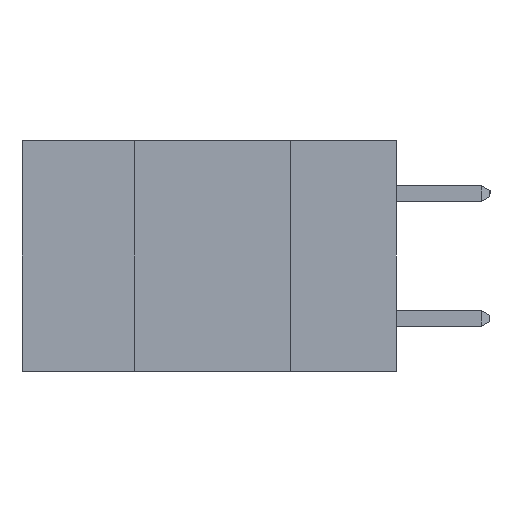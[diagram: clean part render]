
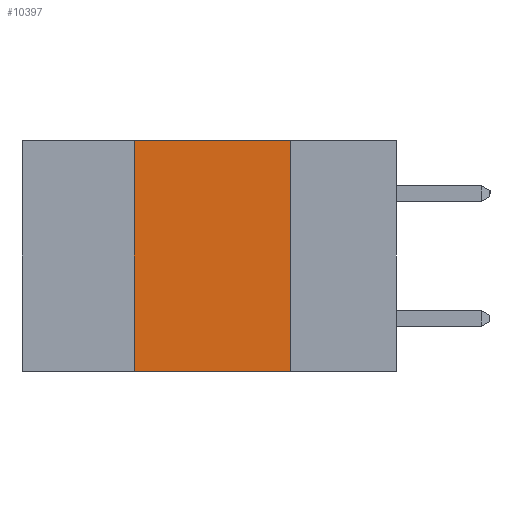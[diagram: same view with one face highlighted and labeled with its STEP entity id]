
A CAD part, left-side view. The second image highlights one B-rep face of the part: STEP entity #10397.
In plain terms, the highlighted planar face has unit normal (-1, 0, 0).
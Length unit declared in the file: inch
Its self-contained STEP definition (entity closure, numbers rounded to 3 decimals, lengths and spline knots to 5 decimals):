
#1438 = PLANE ( 'NONE',  #9139 ) ;
#1587 = EDGE_CURVE ( 'NONE', #10237, #1676, #16990, .T. ) ;
#1663 = FACE_OUTER_BOUND ( 'NONE', #21955, .T. ) ;
#1676 = VERTEX_POINT ( 'NONE', #15715 ) ;
#2738 = ORIENTED_EDGE ( 'NONE', *, *, #1587, .F. ) ;
#3343 = CARTESIAN_POINT ( 'NONE',  ( 0., 0.42, -0.37 ) ) ;
#3896 = VECTOR ( 'NONE', #15156, 39.37008 ) ;
#4046 = VECTOR ( 'NONE', #12525, 39.37008 ) ;
#5323 = CARTESIAN_POINT ( 'NONE',  ( 0., 0.42, -0.37 ) ) ;
#5791 = ORIENTED_EDGE ( 'NONE', *, *, #12398, .T. ) ;
#6889 = DIRECTION ( 'NONE',  ( 0., 0., -1. ) ) ;
#7062 = LINE ( 'NONE', #20868, #15044 ) ;
#9139 = AXIS2_PLACEMENT_3D ( 'NONE', #13674, #20622, #12183 ) ;
#9713 = VERTEX_POINT ( 'NONE', #3343 ) ;
#10237 = VERTEX_POINT ( 'NONE', #16643 ) ;
#10352 = VECTOR ( 'NONE', #6889, 39.37008 ) ;
#10397 = ADVANCED_FACE ( 'NONE', ( #1663 ), #1438, .F. ) ;
#10535 = EDGE_CURVE ( 'NONE', #9713, #10237, #21077, .T. ) ;
#12183 = DIRECTION ( 'NONE',  ( 0., 0., -1. ) ) ;
#12398 = EDGE_CURVE ( 'NONE', #9713, #13122, #7062, .T. ) ;
#12425 = DIRECTION ( 'NONE',  ( 0., -1., 0. ) ) ;
#12525 = DIRECTION ( 'NONE',  ( 0., 0., 1. ) ) ;
#13122 = VERTEX_POINT ( 'NONE', #19873 ) ;
#13674 = CARTESIAN_POINT ( 'NONE',  ( 0., 0.6, 0. ) ) ;
#14467 = EDGE_CURVE ( 'NONE', #1676, #13122, #20690, .T. ) ;
#15044 = VECTOR ( 'NONE', #12425, 39.37008 ) ;
#15156 = DIRECTION ( 'NONE',  ( 0., -1., 0. ) ) ;
#15715 = CARTESIAN_POINT ( 'NONE',  ( 0., 0.17, 0. ) ) ;
#16643 = CARTESIAN_POINT ( 'NONE',  ( 0., 0.42, 0. ) ) ;
#16990 = LINE ( 'NONE', #20621, #3896 ) ;
#19873 = CARTESIAN_POINT ( 'NONE',  ( 0., 0.17, -0.37 ) ) ;
#20485 = ORIENTED_EDGE ( 'NONE', *, *, #14467, .F. ) ;
#20621 = CARTESIAN_POINT ( 'NONE',  ( 0., 0.6, 0. ) ) ;
#20622 = DIRECTION ( 'NONE',  ( 1., 0., 0. ) ) ;
#20690 = LINE ( 'NONE', #22544, #10352 ) ;
#20868 = CARTESIAN_POINT ( 'NONE',  ( 0., 0.6, -0.37 ) ) ;
#21054 = ORIENTED_EDGE ( 'NONE', *, *, #10535, .F. ) ;
#21077 = LINE ( 'NONE', #5323, #4046 ) ;
#21955 = EDGE_LOOP ( 'NONE', ( #20485, #2738, #21054, #5791 ) ) ;
#22544 = CARTESIAN_POINT ( 'NONE',  ( 0., 0.17, -0.37 ) ) ;
